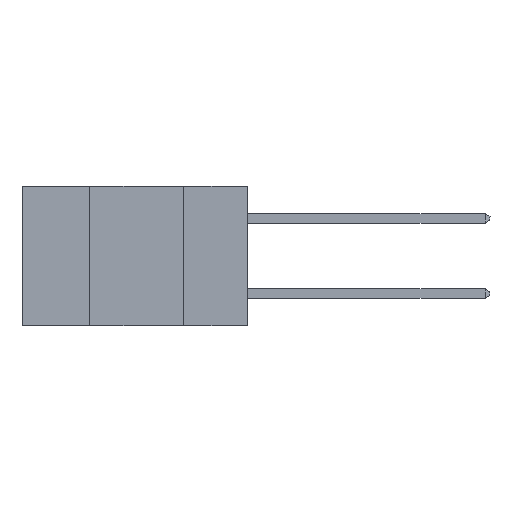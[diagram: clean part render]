
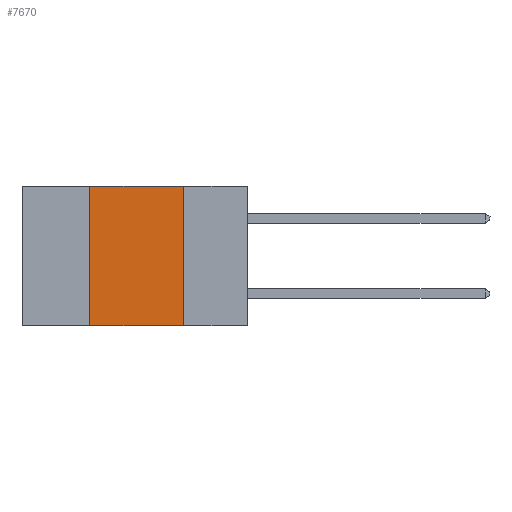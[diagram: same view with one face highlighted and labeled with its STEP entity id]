
A CAD part, left-side view. The second image highlights one B-rep face of the part: STEP entity #7670.
In plain terms, the highlighted planar face has unit normal (-1, 0, 0).
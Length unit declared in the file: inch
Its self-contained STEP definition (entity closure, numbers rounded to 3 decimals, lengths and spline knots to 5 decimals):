
#102 = LINE ( 'NONE', #6496, #2770 ) ;
#382 = EDGE_LOOP ( 'NONE', ( #2577, #5870, #7414, #7895 ) ) ;
#577 = CARTESIAN_POINT ( 'NONE',  ( 0., 0.17, 0. ) ) ;
#580 = EDGE_CURVE ( 'NONE', #2640, #4397, #923, .T. ) ;
#923 = LINE ( 'NONE', #6417, #9032 ) ;
#1282 = LINE ( 'NONE', #9919, #3136 ) ;
#1460 = LINE ( 'NONE', #5338, #5397 ) ;
#1766 = VERTEX_POINT ( 'NONE', #3780 ) ;
#2577 = ORIENTED_EDGE ( 'NONE', *, *, #580, .F. ) ;
#2640 = VERTEX_POINT ( 'NONE', #577 ) ;
#2770 = VECTOR ( 'NONE', #4089, 39.37008 ) ;
#3000 = CARTESIAN_POINT ( 'NONE',  ( 0., 0.17, -0.37 ) ) ;
#3136 = VECTOR ( 'NONE', #5951, 39.37008 ) ;
#3188 = CARTESIAN_POINT ( 'NONE',  ( 0., 0.42, -0.37 ) ) ;
#3666 = AXIS2_PLACEMENT_3D ( 'NONE', #6987, #7808, #10135 ) ;
#3780 = CARTESIAN_POINT ( 'NONE',  ( 0., 0.42, 0. ) ) ;
#3892 = EDGE_CURVE ( 'NONE', #1766, #2640, #1460, .T. ) ;
#4089 = DIRECTION ( 'NONE',  ( 0., 0., 1. ) ) ;
#4397 = VERTEX_POINT ( 'NONE', #3000 ) ;
#4857 = VERTEX_POINT ( 'NONE', #3188 ) ;
#5236 = EDGE_CURVE ( 'NONE', #4857, #1766, #102, .T. ) ;
#5338 = CARTESIAN_POINT ( 'NONE',  ( 0., 0.6, 0. ) ) ;
#5397 = VECTOR ( 'NONE', #6283, 39.37008 ) ;
#5870 = ORIENTED_EDGE ( 'NONE', *, *, #3892, .F. ) ;
#5951 = DIRECTION ( 'NONE',  ( 0., -1., 0. ) ) ;
#6283 = DIRECTION ( 'NONE',  ( 0., -1., 0. ) ) ;
#6417 = CARTESIAN_POINT ( 'NONE',  ( 0., 0.17, -0.37 ) ) ;
#6496 = CARTESIAN_POINT ( 'NONE',  ( 0., 0.42, -0.37 ) ) ;
#6987 = CARTESIAN_POINT ( 'NONE',  ( 0., 0.6, 0. ) ) ;
#7414 = ORIENTED_EDGE ( 'NONE', *, *, #5236, .F. ) ;
#7595 = EDGE_CURVE ( 'NONE', #4857, #4397, #1282, .T. ) ;
#7650 = PLANE ( 'NONE',  #3666 ) ;
#7670 = ADVANCED_FACE ( 'NONE', ( #9198 ), #7650, .F. ) ;
#7808 = DIRECTION ( 'NONE',  ( 1., 0., 0. ) ) ;
#7895 = ORIENTED_EDGE ( 'NONE', *, *, #7595, .T. ) ;
#9032 = VECTOR ( 'NONE', #9550, 39.37008 ) ;
#9198 = FACE_OUTER_BOUND ( 'NONE', #382, .T. ) ;
#9550 = DIRECTION ( 'NONE',  ( 0., 0., -1. ) ) ;
#9919 = CARTESIAN_POINT ( 'NONE',  ( 0., 0.6, -0.37 ) ) ;
#10135 = DIRECTION ( 'NONE',  ( 0., 0., -1. ) ) ;
